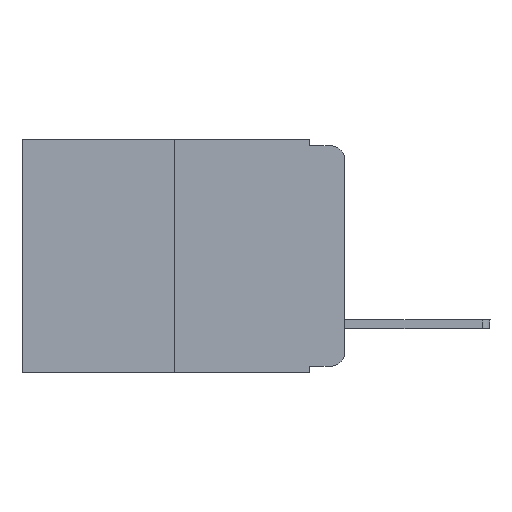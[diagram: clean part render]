
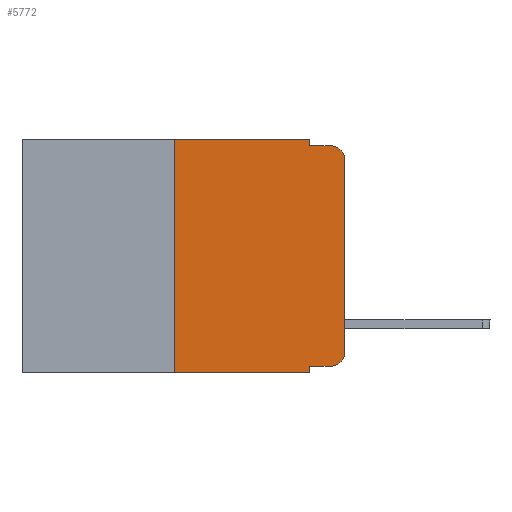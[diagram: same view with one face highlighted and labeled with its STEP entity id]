
A CAD part, left-side view. The second image highlights one B-rep face of the part: STEP entity #5772.
In plain terms, the highlighted planar face has unit normal (-1, 0, 0).
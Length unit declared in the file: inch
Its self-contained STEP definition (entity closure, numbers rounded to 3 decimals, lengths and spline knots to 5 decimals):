
#72 = VECTOR ( 'NONE', #11439, 39.37008 ) ;
#841 = LINE ( 'NONE', #10483, #1078 ) ;
#933 = EDGE_CURVE ( 'NONE', #8305, #3696, #4798, .T. ) ;
#1002 = VECTOR ( 'NONE', #3726, 39.37008 ) ;
#1028 = CARTESIAN_POINT ( 'NONE',  ( 0., 0.473, 0. ) ) ;
#1078 = VECTOR ( 'NONE', #4291, 39.37008 ) ;
#1261 = VECTOR ( 'NONE', #3089, 39.37008 ) ;
#1307 = EDGE_CURVE ( 'NONE', #5330, #4362, #2717, .T. ) ;
#1788 = AXIS2_PLACEMENT_3D ( 'NONE', #10478, #8236, #10624 ) ;
#1887 = FACE_OUTER_BOUND ( 'NONE', #3991, .T. ) ;
#2075 = VERTEX_POINT ( 'NONE', #13072 ) ;
#2624 = CARTESIAN_POINT ( 'NONE',  ( 0., 0.051, -0.01 ) ) ;
#2717 = LINE ( 'NONE', #7150, #72 ) ;
#2971 = CARTESIAN_POINT ( 'NONE',  ( 0., 0.051, -0.333 ) ) ;
#2993 = CARTESIAN_POINT ( 'NONE',  ( 0., 0., -0.313 ) ) ;
#3089 = DIRECTION ( 'NONE',  ( 0., -1., 0. ) ) ;
#3362 = CIRCLE ( 'NONE', #1788, 0.02 ) ;
#3696 = VERTEX_POINT ( 'NONE', #13188 ) ;
#3726 = DIRECTION ( 'NONE',  ( 0., -1., 0. ) ) ;
#3979 = EDGE_CURVE ( 'NONE', #13306, #10042, #841, .T. ) ;
#3991 = EDGE_LOOP ( 'NONE', ( #8407, #8572, #9900, #10452, #6906, #5678, #11605, #10458, #9151, #9207 ) ) ;
#4010 = AXIS2_PLACEMENT_3D ( 'NONE', #1028, #5345, #4077 ) ;
#4077 = DIRECTION ( 'NONE',  ( 0., 0., -1. ) ) ;
#4291 = DIRECTION ( 'NONE',  ( 0., 0., 1. ) ) ;
#4362 = VERTEX_POINT ( 'NONE', #13433 ) ;
#4759 = VECTOR ( 'NONE', #4929, 39.37008 ) ;
#4798 = LINE ( 'NONE', #4940, #8162 ) ;
#4827 = CARTESIAN_POINT ( 'NONE',  ( 0., 0.02, -0.01 ) ) ;
#4929 = DIRECTION ( 'NONE',  ( 0., -1., 0. ) ) ;
#4940 = CARTESIAN_POINT ( 'NONE',  ( 0., 0.25, 0. ) ) ;
#5330 = VERTEX_POINT ( 'NONE', #2971 ) ;
#5345 = DIRECTION ( 'NONE',  ( 1., 0., 0. ) ) ;
#5678 = ORIENTED_EDGE ( 'NONE', *, *, #933, .F. ) ;
#5772 = ADVANCED_FACE ( 'NONE', ( #1887 ), #10677, .F. ) ;
#6027 = VERTEX_POINT ( 'NONE', #12372 ) ;
#6171 = CARTESIAN_POINT ( 'NONE',  ( 0., 0., -0.03 ) ) ;
#6906 = ORIENTED_EDGE ( 'NONE', *, *, #8437, .F. ) ;
#6980 = DIRECTION ( 'NONE',  ( 0., 0., 1. ) ) ;
#7057 = EDGE_CURVE ( 'NONE', #6027, #13306, #3362, .T. ) ;
#7150 = CARTESIAN_POINT ( 'NONE',  ( 0., 0.051, 0. ) ) ;
#7333 = LINE ( 'NONE', #12629, #8674 ) ;
#7386 = CARTESIAN_POINT ( 'NONE',  ( 0., 0.02, -0.03 ) ) ;
#7531 = CARTESIAN_POINT ( 'NONE',  ( 0., 0.25, -0.343 ) ) ;
#7619 = VERTEX_POINT ( 'NONE', #9054 ) ;
#7883 = CARTESIAN_POINT ( 'NONE',  ( 0., 0.473, 0. ) ) ;
#8162 = VECTOR ( 'NONE', #6980, 39.37008 ) ;
#8236 = DIRECTION ( 'NONE',  ( -1., 0., 0. ) ) ;
#8305 = VERTEX_POINT ( 'NONE', #7531 ) ;
#8407 = ORIENTED_EDGE ( 'NONE', *, *, #3979, .T. ) ;
#8437 = EDGE_CURVE ( 'NONE', #3696, #7619, #13382, .T. ) ;
#8572 = ORIENTED_EDGE ( 'NONE', *, *, #9917, .T. ) ;
#8674 = VECTOR ( 'NONE', #12411, 39.37008 ) ;
#9054 = CARTESIAN_POINT ( 'NONE',  ( 0., 0.051, 0. ) ) ;
#9151 = ORIENTED_EDGE ( 'NONE', *, *, #11204, .T. ) ;
#9207 = ORIENTED_EDGE ( 'NONE', *, *, #7057, .T. ) ;
#9503 = LINE ( 'NONE', #11891, #1261 ) ;
#9830 = EDGE_CURVE ( 'NONE', #8305, #4362, #11179, .T. ) ;
#9900 = ORIENTED_EDGE ( 'NONE', *, *, #10405, .F. ) ;
#9917 = EDGE_CURVE ( 'NONE', #10042, #10039, #11129, .T. ) ;
#10039 = VERTEX_POINT ( 'NONE', #4827 ) ;
#10042 = VERTEX_POINT ( 'NONE', #6171 ) ;
#10151 = DIRECTION ( 'NONE',  ( 0., -1., 0. ) ) ;
#10405 = EDGE_CURVE ( 'NONE', #2075, #10039, #12201, .T. ) ;
#10452 = ORIENTED_EDGE ( 'NONE', *, *, #10657, .F. ) ;
#10458 = ORIENTED_EDGE ( 'NONE', *, *, #1307, .F. ) ;
#10478 = CARTESIAN_POINT ( 'NONE',  ( 0., 0.02, -0.313 ) ) ;
#10483 = CARTESIAN_POINT ( 'NONE',  ( 0., 0., 0. ) ) ;
#10624 = DIRECTION ( 'NONE',  ( 0., 0., -1. ) ) ;
#10657 = EDGE_CURVE ( 'NONE', #7619, #2075, #7333, .T. ) ;
#10677 = PLANE ( 'NONE',  #4010 ) ;
#11129 = CIRCLE ( 'NONE', #13626, 0.02 ) ;
#11179 = LINE ( 'NONE', #13385, #1002 ) ;
#11204 = EDGE_CURVE ( 'NONE', #5330, #6027, #9503, .T. ) ;
#11439 = DIRECTION ( 'NONE',  ( 0., 0., -1. ) ) ;
#11605 = ORIENTED_EDGE ( 'NONE', *, *, #9830, .T. ) ;
#11675 = DIRECTION ( 'NONE',  ( 0., 0., -1. ) ) ;
#11891 = CARTESIAN_POINT ( 'NONE',  ( 0., 0.051, -0.333 ) ) ;
#12201 = LINE ( 'NONE', #2624, #12955 ) ;
#12372 = CARTESIAN_POINT ( 'NONE',  ( 0., 0.02, -0.333 ) ) ;
#12411 = DIRECTION ( 'NONE',  ( 0., 0., -1. ) ) ;
#12605 = DIRECTION ( 'NONE',  ( -1., 0., 0. ) ) ;
#12629 = CARTESIAN_POINT ( 'NONE',  ( 0., 0.051, 0. ) ) ;
#12955 = VECTOR ( 'NONE', #10151, 39.37008 ) ;
#13072 = CARTESIAN_POINT ( 'NONE',  ( 0., 0.051, -0.01 ) ) ;
#13188 = CARTESIAN_POINT ( 'NONE',  ( 0., 0.25, 0. ) ) ;
#13306 = VERTEX_POINT ( 'NONE', #2993 ) ;
#13382 = LINE ( 'NONE', #7883, #4759 ) ;
#13385 = CARTESIAN_POINT ( 'NONE',  ( 0., 0.473, -0.343 ) ) ;
#13433 = CARTESIAN_POINT ( 'NONE',  ( 0., 0.051, -0.343 ) ) ;
#13626 = AXIS2_PLACEMENT_3D ( 'NONE', #7386, #12605, #11675 ) ;
